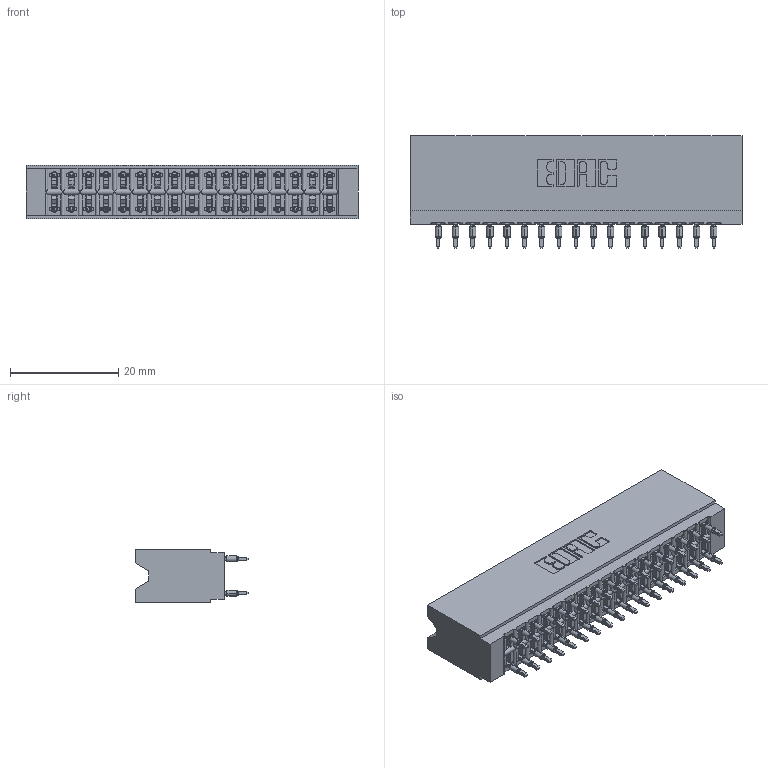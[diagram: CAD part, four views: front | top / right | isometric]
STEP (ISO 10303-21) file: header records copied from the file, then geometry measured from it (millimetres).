
FILE_DESCRIPTION (( 'STEP AP203' ), '1' );
FILE_NAME ('746-034-560-206.STEP', '2026-02-27T00:34:18', ( '' ), ( '' ), 'SwSTEP 2.0', 'SolidWorks 2023', '' );
FILE_SCHEMA (( 'CONFIG_CONTROL_DESIGN' ));
Length unit declared in the file: millimetre
Products named in the file (3): 746-292-001_560; 746 Part_.515 Slot Depth - 06; 746-034-560-206
Assembly tree (35 placements, depth 2):
  746-034-560-206
    746 Part_.515 Slot Depth - 06
    746-292-001_560  x34
Bounding box: 61.21 x 20.82 x 9.91 mm (x, y, z)
Volume: 6817.3 mm3; surface area: 11017.9 mm2
Topology: 35 solids, 35 shells, 3311 faces, 9207 edges, 5904 vertices
Faces by surface type: plane 1654, cylinder 773, bspline 680, torus 204
Entity records: 29970 total; most frequent: CARTESIAN_POINT 6172, ORIENTED_EDGE 5082, DIRECTION 4293, EDGE_CURVE 2541, VECTOR 2179, LINE 2179, VERTEX_POINT 1680, AXIS2_PLACEMENT_3D 1057
